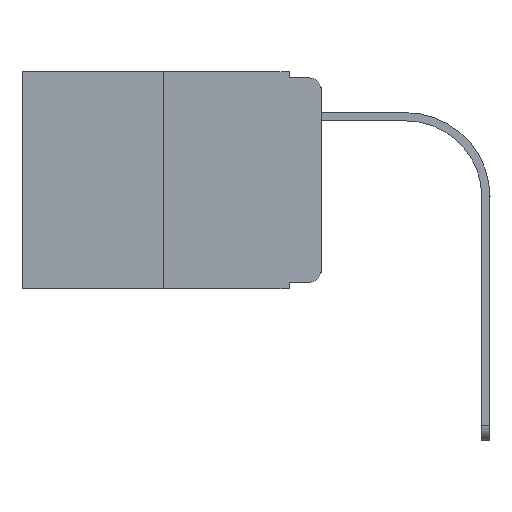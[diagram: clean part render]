
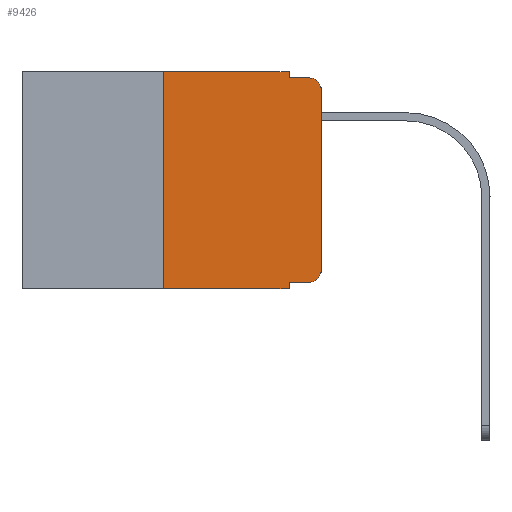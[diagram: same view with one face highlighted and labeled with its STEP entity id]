
A CAD part, left-side view. The second image highlights one B-rep face of the part: STEP entity #9426.
In plain terms, the highlighted planar face has unit normal (-1, 0, 0).
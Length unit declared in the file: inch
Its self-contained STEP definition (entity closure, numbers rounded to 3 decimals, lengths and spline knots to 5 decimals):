
#320 = ORIENTED_EDGE ( 'NONE', *, *, #6925, .F. ) ;
#516 = EDGE_CURVE ( 'NONE', #6380, #22539, #21223, .T. ) ;
#547 = LINE ( 'NONE', #6064, #9978 ) ;
#647 = ORIENTED_EDGE ( 'NONE', *, *, #16093, .T. ) ;
#772 = ORIENTED_EDGE ( 'NONE', *, *, #14524, .T. ) ;
#1448 = EDGE_CURVE ( 'NONE', #3566, #7515, #7543, .T. ) ;
#1635 = DIRECTION ( 'NONE',  ( 0., 0., -1. ) ) ;
#1845 = VECTOR ( 'NONE', #20998, 39.37008 ) ;
#2061 = LINE ( 'NONE', #2171, #19017 ) ;
#2171 = CARTESIAN_POINT ( 'NONE',  ( 0., 0.051, 0. ) ) ;
#2460 = LINE ( 'NONE', #22005, #18433 ) ;
#2625 = CIRCLE ( 'NONE', #16630, 0.02 ) ;
#2751 = DIRECTION ( 'NONE',  ( 0., 0., -1. ) ) ;
#2886 = CARTESIAN_POINT ( 'NONE',  ( 0., 0.02, -0.01 ) ) ;
#3508 = EDGE_CURVE ( 'NONE', #22539, #24657, #7512, .T. ) ;
#3536 = VERTEX_POINT ( 'NONE', #22802 ) ;
#3566 = VERTEX_POINT ( 'NONE', #18650 ) ;
#3839 = EDGE_CURVE ( 'NONE', #3536, #7773, #14011, .T. ) ;
#5258 = VECTOR ( 'NONE', #20241, 39.37008 ) ;
#5426 = EDGE_CURVE ( 'NONE', #3536, #13059, #547, .T. ) ;
#5474 = DIRECTION ( 'NONE',  ( 0., 0., 1. ) ) ;
#6064 = CARTESIAN_POINT ( 'NONE',  ( 0., 0.25, 0. ) ) ;
#6380 = VERTEX_POINT ( 'NONE', #8289 ) ;
#6613 = DIRECTION ( 'NONE',  ( -1., 0., 0. ) ) ;
#6744 = CARTESIAN_POINT ( 'NONE',  ( 0., 0.051, -0.343 ) ) ;
#6925 = EDGE_CURVE ( 'NONE', #22574, #7773, #2061, .T. ) ;
#7512 = LINE ( 'NONE', #18786, #8785 ) ;
#7515 = VERTEX_POINT ( 'NONE', #19543 ) ;
#7543 = LINE ( 'NONE', #15025, #21887 ) ;
#7773 = VERTEX_POINT ( 'NONE', #6744 ) ;
#8226 = DIRECTION ( 'NONE',  ( 0., -1., 0. ) ) ;
#8289 = CARTESIAN_POINT ( 'NONE',  ( 0., 0.02, -0.333 ) ) ;
#8436 = DIRECTION ( 'NONE',  ( -1., 0., 0. ) ) ;
#8639 = CARTESIAN_POINT ( 'NONE',  ( 0., 0.02, -0.313 ) ) ;
#8737 = DIRECTION ( 'NONE',  ( 1., 0., 0. ) ) ;
#8785 = VECTOR ( 'NONE', #5474, 39.37008 ) ;
#8935 = CARTESIAN_POINT ( 'NONE',  ( 0., 0.25, 0. ) ) ;
#9426 = ADVANCED_FACE ( 'NONE', ( #20006 ), #15993, .F. ) ;
#9747 = LINE ( 'NONE', #17639, #1845 ) ;
#9948 = CARTESIAN_POINT ( 'NONE',  ( 0., 0.02, -0.03 ) ) ;
#9978 = VECTOR ( 'NONE', #20981, 39.37008 ) ;
#10182 = DIRECTION ( 'NONE',  ( 0., 0., -1. ) ) ;
#10478 = ORIENTED_EDGE ( 'NONE', *, *, #3508, .T. ) ;
#11121 = ORIENTED_EDGE ( 'NONE', *, *, #19710, .F. ) ;
#11672 = VERTEX_POINT ( 'NONE', #2886 ) ;
#12606 = DIRECTION ( 'NONE',  ( 0., 0., -1. ) ) ;
#13059 = VERTEX_POINT ( 'NONE', #8935 ) ;
#13579 = EDGE_CURVE ( 'NONE', #13059, #3566, #9747, .T. ) ;
#14011 = LINE ( 'NONE', #16244, #5258 ) ;
#14283 = ORIENTED_EDGE ( 'NONE', *, *, #13579, .F. ) ;
#14524 = EDGE_CURVE ( 'NONE', #24657, #11672, #2625, .T. ) ;
#14614 = CARTESIAN_POINT ( 'NONE',  ( 0., 0., -0.03 ) ) ;
#14957 = ORIENTED_EDGE ( 'NONE', *, *, #1448, .F. ) ;
#15025 = CARTESIAN_POINT ( 'NONE',  ( 0., 0.051, 0. ) ) ;
#15618 = AXIS2_PLACEMENT_3D ( 'NONE', #8639, #6613, #2751 ) ;
#15642 = CARTESIAN_POINT ( 'NONE',  ( 0., 0.051, -0.333 ) ) ;
#15993 = PLANE ( 'NONE',  #19138 ) ;
#16093 = EDGE_CURVE ( 'NONE', #22574, #6380, #17402, .T. ) ;
#16244 = CARTESIAN_POINT ( 'NONE',  ( 0., 0.473, -0.343 ) ) ;
#16630 = AXIS2_PLACEMENT_3D ( 'NONE', #9948, #8436, #10182 ) ;
#17402 = LINE ( 'NONE', #15642, #18719 ) ;
#17617 = CARTESIAN_POINT ( 'NONE',  ( 0., 0., -0.313 ) ) ;
#17639 = CARTESIAN_POINT ( 'NONE',  ( 0., 0.473, 0. ) ) ;
#18433 = VECTOR ( 'NONE', #8226, 39.37008 ) ;
#18650 = CARTESIAN_POINT ( 'NONE',  ( 0., 0.051, 0. ) ) ;
#18719 = VECTOR ( 'NONE', #21162, 39.37008 ) ;
#18786 = CARTESIAN_POINT ( 'NONE',  ( 0., 0., 0. ) ) ;
#19017 = VECTOR ( 'NONE', #21240, 39.37008 ) ;
#19138 = AXIS2_PLACEMENT_3D ( 'NONE', #23907, #8737, #12606 ) ;
#19543 = CARTESIAN_POINT ( 'NONE',  ( 0., 0.051, -0.01 ) ) ;
#19710 = EDGE_CURVE ( 'NONE', #7515, #11672, #2460, .T. ) ;
#20006 = FACE_OUTER_BOUND ( 'NONE', #20487, .T. ) ;
#20241 = DIRECTION ( 'NONE',  ( 0., -1., 0. ) ) ;
#20487 = EDGE_LOOP ( 'NONE', ( #10478, #772, #11121, #14957, #14283, #22159, #24093, #320, #647, #24056 ) ) ;
#20981 = DIRECTION ( 'NONE',  ( 0., 0., 1. ) ) ;
#20998 = DIRECTION ( 'NONE',  ( 0., -1., 0. ) ) ;
#21162 = DIRECTION ( 'NONE',  ( 0., -1., 0. ) ) ;
#21223 = CIRCLE ( 'NONE', #15618, 0.02 ) ;
#21240 = DIRECTION ( 'NONE',  ( 0., 0., -1. ) ) ;
#21349 = CARTESIAN_POINT ( 'NONE',  ( 0., 0.051, -0.333 ) ) ;
#21887 = VECTOR ( 'NONE', #1635, 39.37008 ) ;
#22005 = CARTESIAN_POINT ( 'NONE',  ( 0., 0.051, -0.01 ) ) ;
#22159 = ORIENTED_EDGE ( 'NONE', *, *, #5426, .F. ) ;
#22539 = VERTEX_POINT ( 'NONE', #17617 ) ;
#22574 = VERTEX_POINT ( 'NONE', #21349 ) ;
#22802 = CARTESIAN_POINT ( 'NONE',  ( 0., 0.25, -0.343 ) ) ;
#23907 = CARTESIAN_POINT ( 'NONE',  ( 0., 0.473, 0. ) ) ;
#24056 = ORIENTED_EDGE ( 'NONE', *, *, #516, .T. ) ;
#24093 = ORIENTED_EDGE ( 'NONE', *, *, #3839, .T. ) ;
#24657 = VERTEX_POINT ( 'NONE', #14614 ) ;
